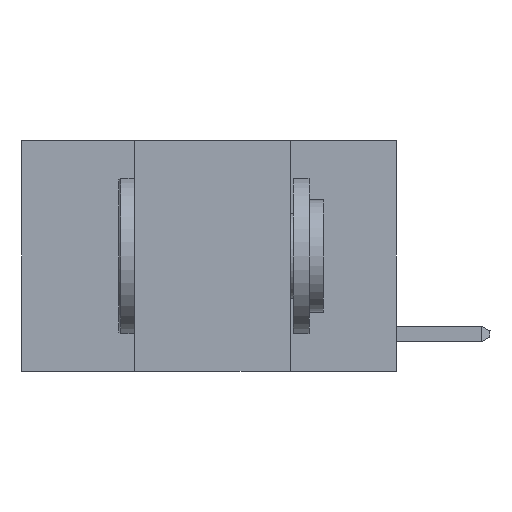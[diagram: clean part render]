
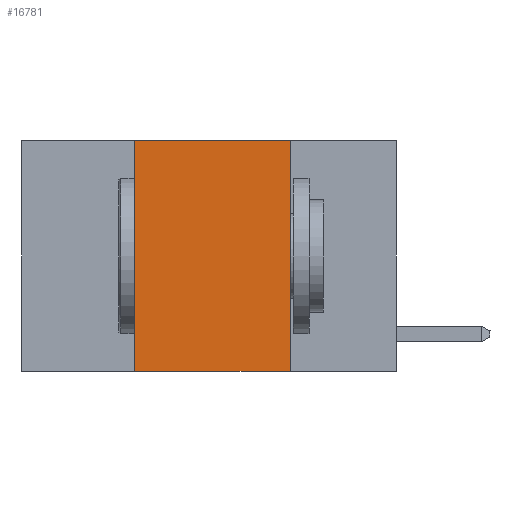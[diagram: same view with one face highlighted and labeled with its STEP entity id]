
A CAD part, left-side view. The second image highlights one B-rep face of the part: STEP entity #16781.
In plain terms, the highlighted planar face has unit normal (-1, 0, 0).
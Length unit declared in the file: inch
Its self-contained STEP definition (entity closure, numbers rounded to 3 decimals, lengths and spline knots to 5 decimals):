
#1170 = CARTESIAN_POINT ( 'NONE',  ( 0., 0.6, 0. ) ) ;
#1191 = EDGE_CURVE ( 'NONE', #14702, #14297, #13949, .T. ) ;
#1595 = ORIENTED_EDGE ( 'NONE', *, *, #5950, .F. ) ;
#3716 = ORIENTED_EDGE ( 'NONE', *, *, #16363, .T. ) ;
#3814 = DIRECTION ( 'NONE',  ( 0., -1., 0. ) ) ;
#3902 = LINE ( 'NONE', #18474, #7612 ) ;
#4736 = ORIENTED_EDGE ( 'NONE', *, *, #9147, .F. ) ;
#5090 = DIRECTION ( 'NONE',  ( 0., -1., 0. ) ) ;
#5950 = EDGE_CURVE ( 'NONE', #13945, #14702, #12546, .T. ) ;
#6567 = DIRECTION ( 'NONE',  ( 0., 0., -1. ) ) ;
#6795 = FACE_OUTER_BOUND ( 'NONE', #12817, .T. ) ;
#7612 = VECTOR ( 'NONE', #3814, 39.37008 ) ;
#7776 = ORIENTED_EDGE ( 'NONE', *, *, #1191, .F. ) ;
#8212 = DIRECTION ( 'NONE',  ( 0., 0., -1. ) ) ;
#8930 = VECTOR ( 'NONE', #5090, 39.37008 ) ;
#9014 = CARTESIAN_POINT ( 'NONE',  ( 0., 0.17, -0.37 ) ) ;
#9104 = LINE ( 'NONE', #12235, #15612 ) ;
#9147 = EDGE_CURVE ( 'NONE', #14297, #12289, #9104, .T. ) ;
#10134 = CARTESIAN_POINT ( 'NONE',  ( 0., 0.42, 0. ) ) ;
#11248 = AXIS2_PLACEMENT_3D ( 'NONE', #1170, #18180, #8212 ) ;
#11934 = CARTESIAN_POINT ( 'NONE',  ( 0., 0.17, 0. ) ) ;
#12235 = CARTESIAN_POINT ( 'NONE',  ( 0., 0.17, 0. ) ) ;
#12289 = VERTEX_POINT ( 'NONE', #9014 ) ;
#12425 = CARTESIAN_POINT ( 'NONE',  ( 0., 0.42, -0.37 ) ) ;
#12546 = LINE ( 'NONE', #18263, #13131 ) ;
#12817 = EDGE_LOOP ( 'NONE', ( #4736, #7776, #1595, #3716 ) ) ;
#13131 = VECTOR ( 'NONE', #15540, 39.37008 ) ;
#13584 = CARTESIAN_POINT ( 'NONE',  ( 0., 0.6, 0. ) ) ;
#13945 = VERTEX_POINT ( 'NONE', #12425 ) ;
#13949 = LINE ( 'NONE', #13584, #8930 ) ;
#14297 = VERTEX_POINT ( 'NONE', #11934 ) ;
#14702 = VERTEX_POINT ( 'NONE', #10134 ) ;
#15540 = DIRECTION ( 'NONE',  ( 0., 0., 1. ) ) ;
#15612 = VECTOR ( 'NONE', #6567, 39.37008 ) ;
#16363 = EDGE_CURVE ( 'NONE', #13945, #12289, #3902, .T. ) ;
#16704 = PLANE ( 'NONE',  #11248 ) ;
#16781 = ADVANCED_FACE ( 'NONE', ( #6795 ), #16704, .F. ) ;
#18180 = DIRECTION ( 'NONE',  ( 1., 0., 0. ) ) ;
#18263 = CARTESIAN_POINT ( 'NONE',  ( 0., 0.42, 0. ) ) ;
#18474 = CARTESIAN_POINT ( 'NONE',  ( 0., 0.6, -0.37 ) ) ;
